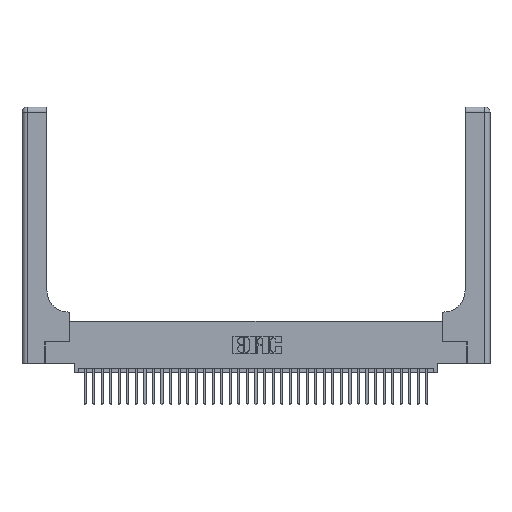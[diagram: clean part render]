
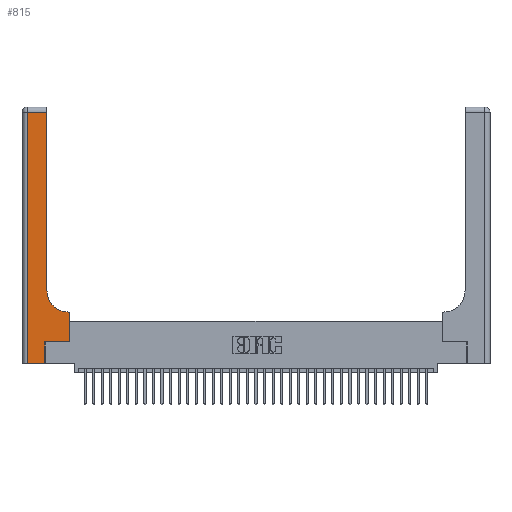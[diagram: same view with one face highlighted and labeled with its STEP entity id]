
A CAD part, top view. The second image highlights one B-rep face of the part: STEP entity #815.
In plain terms, the highlighted planar face has unit normal (0, 0, 1).
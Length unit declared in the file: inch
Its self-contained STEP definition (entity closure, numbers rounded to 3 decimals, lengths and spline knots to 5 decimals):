
#463 = VERTEX_POINT ( 'NONE', #18205 ) ;
#581 = VERTEX_POINT ( 'NONE', #27794 ) ;
#815 = ADVANCED_FACE ( 'NONE', ( #9057 ), #13409, .F. ) ;
#1524 = CARTESIAN_POINT ( 'NONE',  ( 0.5415, 0.6, 0.37 ) ) ;
#2290 = CIRCLE ( 'NONE', #4009, 0.25 ) ;
#2649 = CARTESIAN_POINT ( 'NONE',  ( 0.2915, 2.94, 0.37 ) ) ;
#2767 = CARTESIAN_POINT ( 'NONE',  ( 0., 2.94, 0.37 ) ) ;
#4009 = AXIS2_PLACEMENT_3D ( 'NONE', #29328, #32590, #26561 ) ;
#4768 = DIRECTION ( 'NONE',  ( 0., 0., -1. ) ) ;
#4996 = VECTOR ( 'NONE', #18459, 39.37008 ) ;
#7657 = LINE ( 'NONE', #11744, #37242 ) ;
#7955 = LINE ( 'NONE', #18915, #30668 ) ;
#8114 = CARTESIAN_POINT ( 'NONE',  ( 0.2915, 0.85, 0.37 ) ) ;
#9057 = FACE_OUTER_BOUND ( 'NONE', #24490, .T. ) ;
#9574 = CARTESIAN_POINT ( 'NONE',  ( 0.2915, 0.6, 0.37 ) ) ;
#9636 = EDGE_CURVE ( 'NONE', #12884, #13324, #30789, .T. ) ;
#10414 = ORIENTED_EDGE ( 'NONE', *, *, #15857, .T. ) ;
#11494 = VERTEX_POINT ( 'NONE', #8114 ) ;
#11744 = CARTESIAN_POINT ( 'NONE',  ( 0.06, 3., 0.37 ) ) ;
#12884 = VERTEX_POINT ( 'NONE', #34402 ) ;
#13324 = VERTEX_POINT ( 'NONE', #14431 ) ;
#13409 = PLANE ( 'NONE',  #30873 ) ;
#13525 = DIRECTION ( 'NONE',  ( -1., 0., 0. ) ) ;
#14200 = CARTESIAN_POINT ( 'NONE',  ( 0.269, 0., 0.37 ) ) ;
#14284 = EDGE_CURVE ( 'NONE', #22598, #11494, #2290, .T. ) ;
#14431 = CARTESIAN_POINT ( 'NONE',  ( 0.5585, 0.25, 0.37 ) ) ;
#15027 = LINE ( 'NONE', #2767, #26455 ) ;
#15135 = LINE ( 'NONE', #34603, #33388 ) ;
#15610 = VECTOR ( 'NONE', #18622, 39.37008 ) ;
#15857 = EDGE_CURVE ( 'NONE', #33437, #19504, #15027, .T. ) ;
#15898 = VERTEX_POINT ( 'NONE', #14200 ) ;
#16266 = CARTESIAN_POINT ( 'NONE',  ( 0.269, 0.25, 0.37 ) ) ;
#16309 = ORIENTED_EDGE ( 'NONE', *, *, #29113, .T. ) ;
#18191 = LINE ( 'NONE', #9574, #4996 ) ;
#18205 = CARTESIAN_POINT ( 'NONE',  ( 0.06, 0., 0.37 ) ) ;
#18459 = DIRECTION ( 'NONE',  ( -1., 0., 0. ) ) ;
#18622 = DIRECTION ( 'NONE',  ( 1., 0., 0. ) ) ;
#18915 = CARTESIAN_POINT ( 'NONE',  ( 0.2915, 3., 0.37 ) ) ;
#19075 = DIRECTION ( 'NONE',  ( 1., 0., 0. ) ) ;
#19504 = VERTEX_POINT ( 'NONE', #36123 ) ;
#20077 = DIRECTION ( 'NONE',  ( 0., 1., 0. ) ) ;
#20311 = EDGE_CURVE ( 'NONE', #15898, #12884, #15135, .T. ) ;
#20335 = ORIENTED_EDGE ( 'NONE', *, *, #20311, .T. ) ;
#20594 = ORIENTED_EDGE ( 'NONE', *, *, #29714, .T. ) ;
#21237 = VECTOR ( 'NONE', #19075, 39.37008 ) ;
#22373 = ORIENTED_EDGE ( 'NONE', *, *, #36684, .T. ) ;
#22598 = VERTEX_POINT ( 'NONE', #1524 ) ;
#22973 = DIRECTION ( 'NONE',  ( -1., 0., 0. ) ) ;
#24490 = EDGE_LOOP ( 'NONE', ( #16309, #10414, #25107, #20594, #20335, #31792, #36695, #22373, #31043 ) ) ;
#25107 = ORIENTED_EDGE ( 'NONE', *, *, #32291, .T. ) ;
#26455 = VECTOR ( 'NONE', #22973, 39.37008 ) ;
#26528 = DIRECTION ( 'NONE',  ( 0., -1., 0. ) ) ;
#26561 = DIRECTION ( 'NONE',  ( 1., 0., 0. ) ) ;
#27029 = LINE ( 'NONE', #33118, #15610 ) ;
#27794 = CARTESIAN_POINT ( 'NONE',  ( 0.5585, 0.6, 0.37 ) ) ;
#27836 = DIRECTION ( 'NONE',  ( 0., 1., 0. ) ) ;
#28545 = VECTOR ( 'NONE', #27836, 39.37008 ) ;
#29113 = EDGE_CURVE ( 'NONE', #11494, #33437, #7955, .T. ) ;
#29328 = CARTESIAN_POINT ( 'NONE',  ( 0.5415, 0.85, 0.37 ) ) ;
#29714 = EDGE_CURVE ( 'NONE', #463, #15898, #27029, .T. ) ;
#30668 = VECTOR ( 'NONE', #35853, 39.37008 ) ;
#30789 = LINE ( 'NONE', #16266, #21237 ) ;
#30873 = AXIS2_PLACEMENT_3D ( 'NONE', #36676, #4768, #13525 ) ;
#31043 = ORIENTED_EDGE ( 'NONE', *, *, #14284, .T. ) ;
#31792 = ORIENTED_EDGE ( 'NONE', *, *, #9636, .T. ) ;
#32291 = EDGE_CURVE ( 'NONE', #19504, #463, #7657, .T. ) ;
#32590 = DIRECTION ( 'NONE',  ( 0., 0., -1. ) ) ;
#33118 = CARTESIAN_POINT ( 'NONE',  ( 0., 0., 0.37 ) ) ;
#33234 = EDGE_CURVE ( 'NONE', #13324, #581, #33994, .T. ) ;
#33388 = VECTOR ( 'NONE', #20077, 39.37008 ) ;
#33437 = VERTEX_POINT ( 'NONE', #2649 ) ;
#33795 = CARTESIAN_POINT ( 'NONE',  ( 0.5585, 0.25, 0.37 ) ) ;
#33994 = LINE ( 'NONE', #33795, #28545 ) ;
#34402 = CARTESIAN_POINT ( 'NONE',  ( 0.269, 0.25, 0.37 ) ) ;
#34603 = CARTESIAN_POINT ( 'NONE',  ( 0.269, 0., 0.37 ) ) ;
#35853 = DIRECTION ( 'NONE',  ( 0., 1., 0. ) ) ;
#36123 = CARTESIAN_POINT ( 'NONE',  ( 0.06, 2.94, 0.37 ) ) ;
#36676 = CARTESIAN_POINT ( 'NONE',  ( 0., 3., 0.37 ) ) ;
#36684 = EDGE_CURVE ( 'NONE', #581, #22598, #18191, .T. ) ;
#36695 = ORIENTED_EDGE ( 'NONE', *, *, #33234, .T. ) ;
#37242 = VECTOR ( 'NONE', #26528, 39.37008 ) ;
